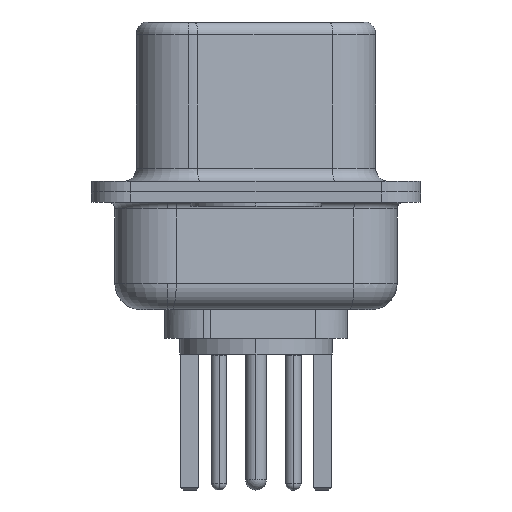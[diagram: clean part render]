
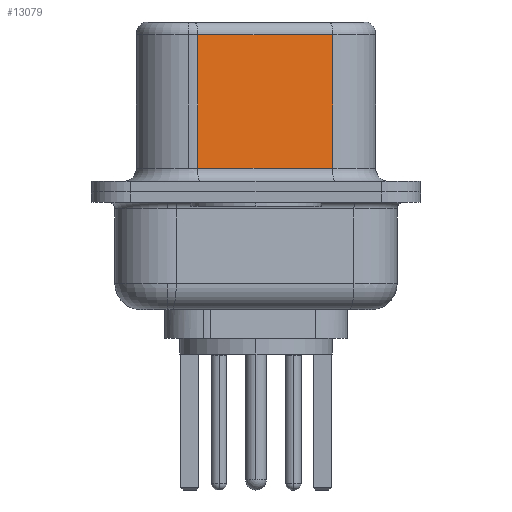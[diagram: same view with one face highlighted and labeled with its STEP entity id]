
A CAD part, left-side view. The second image highlights one B-rep face of the part: STEP entity #13079.
In plain terms, the highlighted planar face has unit normal (-0.985, -0.174, 0).
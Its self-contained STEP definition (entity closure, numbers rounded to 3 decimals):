
#1635 = VECTOR ( 'NONE', #6966, 1000. ) ;
#1682 = LINE ( 'NONE', #10659, #12838 ) ;
#1956 = DIRECTION ( 'NONE',  ( 0., 0., -1. ) ) ;
#2645 = DIRECTION ( 'NONE',  ( 0.985, 0.174, 0. ) ) ;
#2663 = CARTESIAN_POINT ( 'NONE',  ( 4.585, -2.927, 6.02 ) ) ;
#3015 = EDGE_CURVE ( 'NONE', #3369, #10519, #9722, .T. ) ;
#3369 = VERTEX_POINT ( 'NONE', #10415 ) ;
#4790 = VERTEX_POINT ( 'NONE', #2663 ) ;
#5300 = DIRECTION ( 'NONE',  ( -0.174, 0.985, 0. ) ) ;
#5436 = ORIENTED_EDGE ( 'NONE', *, *, #3015, .T. ) ;
#6145 = DIRECTION ( 'NONE',  ( 0., 0., -1. ) ) ;
#6548 = VERTEX_POINT ( 'NONE', #18348 ) ;
#6966 = DIRECTION ( 'NONE',  ( 0.174, -0.985, 0. ) ) ;
#9257 = VECTOR ( 'NONE', #6145, 1000. ) ;
#9722 = LINE ( 'NONE', #18750, #9257 ) ;
#9800 = EDGE_CURVE ( 'NONE', #4790, #6548, #1682, .T. ) ;
#10288 = EDGE_LOOP ( 'NONE', ( #11354, #17931, #5436, #15168 ) ) ;
#10415 = CARTESIAN_POINT ( 'NONE',  ( 3.675, 2.233, 6.02 ) ) ;
#10519 = VERTEX_POINT ( 'NONE', #12423 ) ;
#10659 = CARTESIAN_POINT ( 'NONE',  ( 4.585, -2.927, 6.52 ) ) ;
#11220 = EDGE_CURVE ( 'NONE', #4790, #3369, #17205, .T. ) ;
#11257 = CARTESIAN_POINT ( 'NONE',  ( 4.585, -2.927, 0.9 ) ) ;
#11352 = AXIS2_PLACEMENT_3D ( 'NONE', #18784, #2645, #12835 ) ;
#11354 = ORIENTED_EDGE ( 'NONE', *, *, #9800, .F. ) ;
#12423 = CARTESIAN_POINT ( 'NONE',  ( 3.675, 2.233, 0.9 ) ) ;
#12755 = FACE_OUTER_BOUND ( 'NONE', #10288, .T. ) ;
#12835 = DIRECTION ( 'NONE',  ( -0.174, 0.985, 0. ) ) ;
#12838 = VECTOR ( 'NONE', #1956, 1000. ) ;
#13079 = ADVANCED_FACE ( 'NONE', ( #12755 ), #15671, .F. ) ;
#13240 = VECTOR ( 'NONE', #5300, 1000. ) ;
#13252 = LINE ( 'NONE', #11257, #1635 ) ;
#15168 = ORIENTED_EDGE ( 'NONE', *, *, #17870, .T. ) ;
#15434 = CARTESIAN_POINT ( 'NONE',  ( 4.585, -2.927, 6.02 ) ) ;
#15671 = PLANE ( 'NONE',  #11352 ) ;
#17205 = LINE ( 'NONE', #15434, #13240 ) ;
#17870 = EDGE_CURVE ( 'NONE', #10519, #6548, #13252, .T. ) ;
#17931 = ORIENTED_EDGE ( 'NONE', *, *, #11220, .T. ) ;
#18348 = CARTESIAN_POINT ( 'NONE',  ( 4.585, -2.927, 0.9 ) ) ;
#18750 = CARTESIAN_POINT ( 'NONE',  ( 3.675, 2.233, 6.52 ) ) ;
#18784 = CARTESIAN_POINT ( 'NONE',  ( 4.585, -2.927, 6.52 ) ) ;
